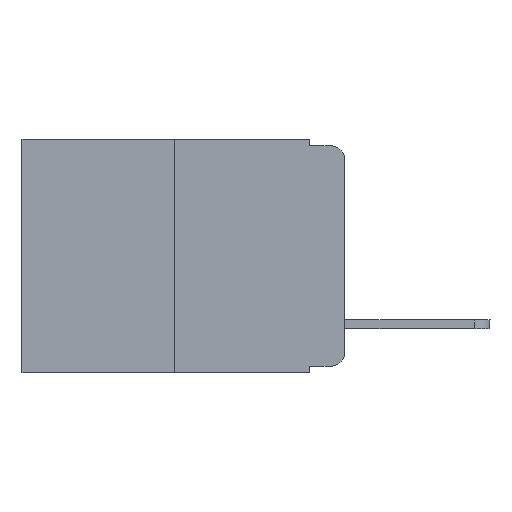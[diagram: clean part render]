
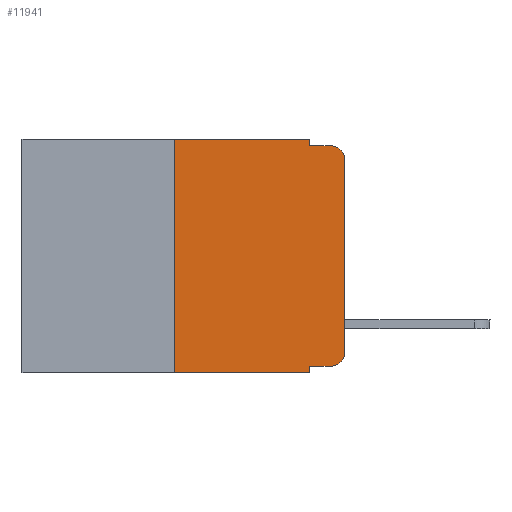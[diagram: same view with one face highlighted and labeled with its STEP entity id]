
A CAD part, left-side view. The second image highlights one B-rep face of the part: STEP entity #11941.
In plain terms, the highlighted planar face has unit normal (-1, 0, 0).
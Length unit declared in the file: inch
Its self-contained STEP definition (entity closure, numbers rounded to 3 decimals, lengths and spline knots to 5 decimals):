
#168 = VECTOR ( 'NONE', #10044, 39.37008 ) ;
#256 = VECTOR ( 'NONE', #2414, 39.37008 ) ;
#263 = CARTESIAN_POINT ( 'NONE',  ( 0., 0.25, -0.343 ) ) ;
#305 = CARTESIAN_POINT ( 'NONE',  ( 0., 0.051, 0. ) ) ;
#312 = EDGE_CURVE ( 'NONE', #9681, #14545, #6003, .T. ) ;
#673 = CARTESIAN_POINT ( 'NONE',  ( 0., 0.051, -0.01 ) ) ;
#785 = ORIENTED_EDGE ( 'NONE', *, *, #12825, .F. ) ;
#1016 = FACE_OUTER_BOUND ( 'NONE', #4406, .T. ) ;
#1086 = VECTOR ( 'NONE', #1231, 39.37008 ) ;
#1231 = DIRECTION ( 'NONE',  ( 0., -1., 0. ) ) ;
#1436 = DIRECTION ( 'NONE',  ( 0., 0., -1. ) ) ;
#1478 = LINE ( 'NONE', #15636, #1086 ) ;
#1525 = DIRECTION ( 'NONE',  ( 0., 0., -1. ) ) ;
#1562 = DIRECTION ( 'NONE',  ( 0., 0., -1. ) ) ;
#1588 = VERTEX_POINT ( 'NONE', #673 ) ;
#1671 = ORIENTED_EDGE ( 'NONE', *, *, #8361, .F. ) ;
#2067 = EDGE_CURVE ( 'NONE', #12993, #2724, #5485, .T. ) ;
#2093 = VECTOR ( 'NONE', #1562, 39.37008 ) ;
#2414 = DIRECTION ( 'NONE',  ( 0., 0., 1. ) ) ;
#2451 = DIRECTION ( 'NONE',  ( 0., 0., -1. ) ) ;
#2724 = VERTEX_POINT ( 'NONE', #10960 ) ;
#2774 = ORIENTED_EDGE ( 'NONE', *, *, #16302, .T. ) ;
#2803 = VERTEX_POINT ( 'NONE', #4344 ) ;
#2982 = LINE ( 'NONE', #5374, #7615 ) ;
#3465 = CARTESIAN_POINT ( 'NONE',  ( 0., 0.02, -0.03 ) ) ;
#3754 = LINE ( 'NONE', #11561, #4621 ) ;
#3787 = CARTESIAN_POINT ( 'NONE',  ( 0., 0.25, 0. ) ) ;
#3871 = DIRECTION ( 'NONE',  ( 0., 0., 1. ) ) ;
#4072 = LINE ( 'NONE', #305, #8994 ) ;
#4185 = ORIENTED_EDGE ( 'NONE', *, *, #4523, .T. ) ;
#4344 = CARTESIAN_POINT ( 'NONE',  ( 0., 0.25, 0. ) ) ;
#4406 = EDGE_LOOP ( 'NONE', ( #9761, #4185, #1671, #12683, #15182, #785, #2774, #15601, #15832, #5513 ) ) ;
#4523 = EDGE_CURVE ( 'NONE', #10912, #14865, #10319, .T. ) ;
#4621 = VECTOR ( 'NONE', #7659, 39.37008 ) ;
#4715 = VECTOR ( 'NONE', #3871, 39.37008 ) ;
#5146 = CARTESIAN_POINT ( 'NONE',  ( 0., 0.02, -0.333 ) ) ;
#5217 = AXIS2_PLACEMENT_3D ( 'NONE', #16640, #10098, #1525 ) ;
#5374 = CARTESIAN_POINT ( 'NONE',  ( 0., 0.473, 0. ) ) ;
#5485 = LINE ( 'NONE', #10554, #2093 ) ;
#5513 = ORIENTED_EDGE ( 'NONE', *, *, #312, .T. ) ;
#5592 = CARTESIAN_POINT ( 'NONE',  ( 0., 0.051, 0. ) ) ;
#5893 = CARTESIAN_POINT ( 'NONE',  ( 0., 0.051, -0.333 ) ) ;
#6003 = CIRCLE ( 'NONE', #10051, 0.02 ) ;
#6219 = PLANE ( 'NONE',  #5217 ) ;
#6236 = CARTESIAN_POINT ( 'NONE',  ( 0., 0.473, -0.343 ) ) ;
#6340 = CARTESIAN_POINT ( 'NONE',  ( 0., 0., 0. ) ) ;
#6503 = LINE ( 'NONE', #6340, #256 ) ;
#7291 = DIRECTION ( 'NONE',  ( -1., 0., 0. ) ) ;
#7606 = EDGE_CURVE ( 'NONE', #12993, #9681, #3754, .T. ) ;
#7615 = VECTOR ( 'NONE', #13107, 39.37008 ) ;
#7659 = DIRECTION ( 'NONE',  ( 0., -1., 0. ) ) ;
#8361 = EDGE_CURVE ( 'NONE', #1588, #14865, #1478, .T. ) ;
#8994 = VECTOR ( 'NONE', #1436, 39.37008 ) ;
#9681 = VERTEX_POINT ( 'NONE', #5146 ) ;
#9722 = EDGE_CURVE ( 'NONE', #14545, #10912, #6503, .T. ) ;
#9761 = ORIENTED_EDGE ( 'NONE', *, *, #9722, .T. ) ;
#9830 = VERTEX_POINT ( 'NONE', #263 ) ;
#9886 = LINE ( 'NONE', #6236, #168 ) ;
#10044 = DIRECTION ( 'NONE',  ( 0., -1., 0. ) ) ;
#10051 = AXIS2_PLACEMENT_3D ( 'NONE', #14196, #11627, #2451 ) ;
#10098 = DIRECTION ( 'NONE',  ( 1., 0., 0. ) ) ;
#10231 = CARTESIAN_POINT ( 'NONE',  ( 0., 0., -0.03 ) ) ;
#10262 = EDGE_CURVE ( 'NONE', #2803, #15542, #2982, .T. ) ;
#10319 = CIRCLE ( 'NONE', #12764, 0.02 ) ;
#10554 = CARTESIAN_POINT ( 'NONE',  ( 0., 0.051, 0. ) ) ;
#10688 = EDGE_CURVE ( 'NONE', #15542, #1588, #4072, .T. ) ;
#10912 = VERTEX_POINT ( 'NONE', #10231 ) ;
#10960 = CARTESIAN_POINT ( 'NONE',  ( 0., 0.051, -0.343 ) ) ;
#11561 = CARTESIAN_POINT ( 'NONE',  ( 0., 0.051, -0.333 ) ) ;
#11627 = DIRECTION ( 'NONE',  ( -1., 0., 0. ) ) ;
#11941 = ADVANCED_FACE ( 'NONE', ( #1016 ), #6219, .F. ) ;
#12573 = CARTESIAN_POINT ( 'NONE',  ( 0., 0.02, -0.01 ) ) ;
#12683 = ORIENTED_EDGE ( 'NONE', *, *, #10688, .F. ) ;
#12764 = AXIS2_PLACEMENT_3D ( 'NONE', #3465, #7291, #13765 ) ;
#12825 = EDGE_CURVE ( 'NONE', #9830, #2803, #14339, .T. ) ;
#12993 = VERTEX_POINT ( 'NONE', #5893 ) ;
#13107 = DIRECTION ( 'NONE',  ( 0., -1., 0. ) ) ;
#13730 = CARTESIAN_POINT ( 'NONE',  ( 0., 0., -0.313 ) ) ;
#13765 = DIRECTION ( 'NONE',  ( 0., 0., -1. ) ) ;
#14196 = CARTESIAN_POINT ( 'NONE',  ( 0., 0.02, -0.313 ) ) ;
#14339 = LINE ( 'NONE', #3787, #4715 ) ;
#14545 = VERTEX_POINT ( 'NONE', #13730 ) ;
#14865 = VERTEX_POINT ( 'NONE', #12573 ) ;
#15182 = ORIENTED_EDGE ( 'NONE', *, *, #10262, .F. ) ;
#15542 = VERTEX_POINT ( 'NONE', #5592 ) ;
#15601 = ORIENTED_EDGE ( 'NONE', *, *, #2067, .F. ) ;
#15636 = CARTESIAN_POINT ( 'NONE',  ( 0., 0.051, -0.01 ) ) ;
#15832 = ORIENTED_EDGE ( 'NONE', *, *, #7606, .T. ) ;
#16302 = EDGE_CURVE ( 'NONE', #9830, #2724, #9886, .T. ) ;
#16640 = CARTESIAN_POINT ( 'NONE',  ( 0., 0.473, 0. ) ) ;
